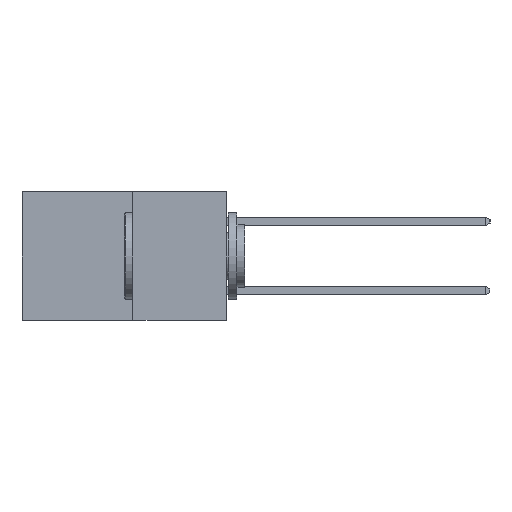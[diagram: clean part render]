
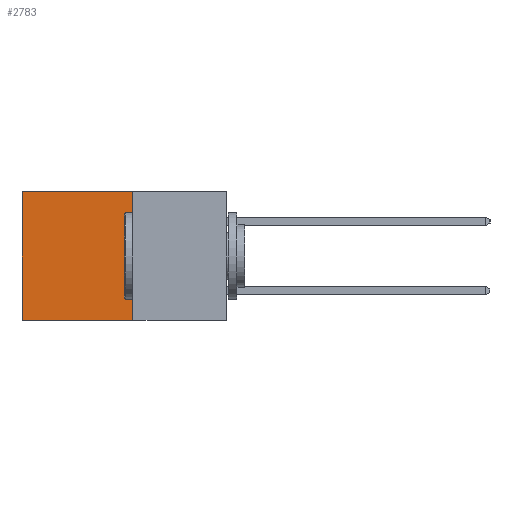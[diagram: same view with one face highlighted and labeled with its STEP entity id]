
A CAD part, left-side view. The second image highlights one B-rep face of the part: STEP entity #2783.
In plain terms, the highlighted planar face has unit normal (-1, 0, 0).
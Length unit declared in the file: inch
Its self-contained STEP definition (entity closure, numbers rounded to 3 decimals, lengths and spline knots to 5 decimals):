
#1570 = AXIS2_PLACEMENT_3D ( 'NONE', #17369, #12263, #14940 ) ;
#1748 = EDGE_CURVE ( 'NONE', #5294, #10093, #12577, .T. ) ;
#2512 = EDGE_CURVE ( 'NONE', #17635, #14870, #7606, .T. ) ;
#2696 = ORIENTED_EDGE ( 'NONE', *, *, #9333, .F. ) ;
#2783 = ADVANCED_FACE ( 'NONE', ( #21085 ), #8616, .F. ) ;
#5294 = VERTEX_POINT ( 'NONE', #5994 ) ;
#5994 = CARTESIAN_POINT ( 'NONE',  ( 0.277, 0.59, 0. ) ) ;
#6543 = VECTOR ( 'NONE', #8846, 39.37008 ) ;
#6941 = CARTESIAN_POINT ( 'NONE',  ( 0.277, 0.27, 0. ) ) ;
#7266 = CARTESIAN_POINT ( 'NONE',  ( 0.277, 0.59, -0.37 ) ) ;
#7322 = EDGE_CURVE ( 'NONE', #17635, #5294, #16220, .T. ) ;
#7606 = LINE ( 'NONE', #19793, #11963 ) ;
#7654 = VECTOR ( 'NONE', #10177, 39.37008 ) ;
#7705 = CARTESIAN_POINT ( 'NONE',  ( 0.277, 0.27, 0. ) ) ;
#8616 = PLANE ( 'NONE',  #1570 ) ;
#8846 = DIRECTION ( 'NONE',  ( 0., 1., 0. ) ) ;
#8897 = ORIENTED_EDGE ( 'NONE', *, *, #2512, .F. ) ;
#9333 = EDGE_CURVE ( 'NONE', #14870, #10093, #18750, .T. ) ;
#10082 = CARTESIAN_POINT ( 'NONE',  ( 0.277, 0.59, -0.37 ) ) ;
#10093 = VERTEX_POINT ( 'NONE', #10082 ) ;
#10177 = DIRECTION ( 'NONE',  ( 0., 0., -1. ) ) ;
#11819 = CARTESIAN_POINT ( 'NONE',  ( 0.277, 0.27, -0.37 ) ) ;
#11963 = VECTOR ( 'NONE', #19766, 39.37008 ) ;
#12263 = DIRECTION ( 'NONE',  ( 1., 0., 0. ) ) ;
#12577 = LINE ( 'NONE', #7266, #7654 ) ;
#13737 = ORIENTED_EDGE ( 'NONE', *, *, #7322, .T. ) ;
#14029 = VECTOR ( 'NONE', #17600, 39.37008 ) ;
#14870 = VERTEX_POINT ( 'NONE', #11819 ) ;
#14940 = DIRECTION ( 'NONE',  ( 0., 0., -1. ) ) ;
#16220 = LINE ( 'NONE', #6941, #6543 ) ;
#17369 = CARTESIAN_POINT ( 'NONE',  ( 0.277, 0.27, -0.37 ) ) ;
#17519 = EDGE_LOOP ( 'NONE', ( #21654, #2696, #8897, #13737 ) ) ;
#17600 = DIRECTION ( 'NONE',  ( 0., 1., 0. ) ) ;
#17635 = VERTEX_POINT ( 'NONE', #7705 ) ;
#18750 = LINE ( 'NONE', #21032, #14029 ) ;
#19766 = DIRECTION ( 'NONE',  ( 0., 0., -1. ) ) ;
#19793 = CARTESIAN_POINT ( 'NONE',  ( 0.277, 0.27, -0.37 ) ) ;
#21032 = CARTESIAN_POINT ( 'NONE',  ( 0.277, 0.27, -0.37 ) ) ;
#21085 = FACE_OUTER_BOUND ( 'NONE', #17519, .T. ) ;
#21654 = ORIENTED_EDGE ( 'NONE', *, *, #1748, .T. ) ;
